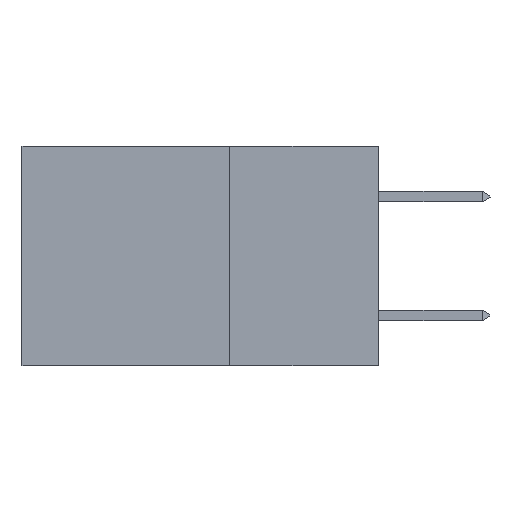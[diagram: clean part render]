
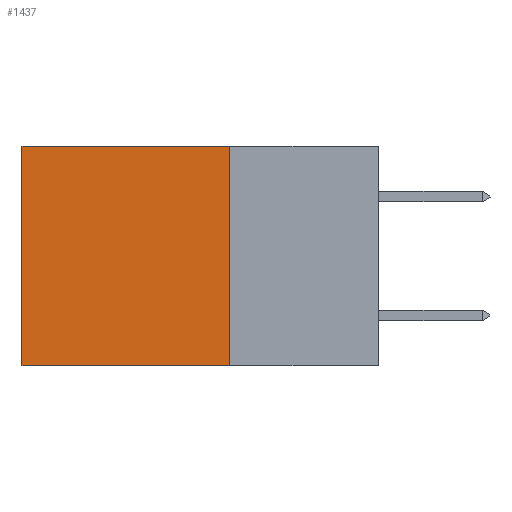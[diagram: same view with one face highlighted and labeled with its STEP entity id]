
A CAD part, left-side view. The second image highlights one B-rep face of the part: STEP entity #1437.
In plain terms, the highlighted planar face has unit normal (-1, 0, 0).
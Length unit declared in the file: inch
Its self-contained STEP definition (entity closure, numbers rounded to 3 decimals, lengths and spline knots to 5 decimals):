
#185 = CARTESIAN_POINT ( 'NONE',  ( 0.298, 0.25, -0.37 ) ) ;
#288 = EDGE_LOOP ( 'NONE', ( #7681, #10519, #3597, #2928 ) ) ;
#947 = DIRECTION ( 'NONE',  ( 1., 0., 0. ) ) ;
#1437 = ADVANCED_FACE ( 'NONE', ( #12549 ), #7735, .F. ) ;
#1477 = EDGE_CURVE ( 'NONE', #9603, #2144, #6084, .T. ) ;
#2076 = CARTESIAN_POINT ( 'NONE',  ( 0.298, 0.25, 0. ) ) ;
#2144 = VERTEX_POINT ( 'NONE', #185 ) ;
#2149 = EDGE_CURVE ( 'NONE', #2144, #10290, #9883, .T. ) ;
#2884 = CARTESIAN_POINT ( 'NONE',  ( 0.298, 0.6, 0. ) ) ;
#2928 = ORIENTED_EDGE ( 'NONE', *, *, #3983, .T. ) ;
#2933 = CARTESIAN_POINT ( 'NONE',  ( 0.298, 0.6, 0. ) ) ;
#3207 = DIRECTION ( 'NONE',  ( 0., 0., -1. ) ) ;
#3597 = ORIENTED_EDGE ( 'NONE', *, *, #1477, .F. ) ;
#3614 = CARTESIAN_POINT ( 'NONE',  ( 0.298, 0.25, 0. ) ) ;
#3936 = VECTOR ( 'NONE', #12483, 39.37008 ) ;
#3954 = CARTESIAN_POINT ( 'NONE',  ( 0.298, 0.6, -0.37 ) ) ;
#3983 = EDGE_CURVE ( 'NONE', #9603, #10098, #11292, .T. ) ;
#4499 = VECTOR ( 'NONE', #12167, 39.37008 ) ;
#4834 = VECTOR ( 'NONE', #7199, 39.37008 ) ;
#5842 = CARTESIAN_POINT ( 'NONE',  ( 0.298, 0.25, -0.37 ) ) ;
#5880 = DIRECTION ( 'NONE',  ( 0., 1., 0. ) ) ;
#6084 = LINE ( 'NONE', #2076, #4499 ) ;
#6552 = CARTESIAN_POINT ( 'NONE',  ( 0.298, 0.25, 0. ) ) ;
#7199 = DIRECTION ( 'NONE',  ( 0., 0., -1. ) ) ;
#7681 = ORIENTED_EDGE ( 'NONE', *, *, #10935, .T. ) ;
#7735 = PLANE ( 'NONE',  #9898 ) ;
#7775 = CARTESIAN_POINT ( 'NONE',  ( 0.298, 0.25, 0. ) ) ;
#9603 = VERTEX_POINT ( 'NONE', #7775 ) ;
#9883 = LINE ( 'NONE', #5842, #3936 ) ;
#9898 = AXIS2_PLACEMENT_3D ( 'NONE', #6552, #947, #3207 ) ;
#10098 = VERTEX_POINT ( 'NONE', #2884 ) ;
#10290 = VERTEX_POINT ( 'NONE', #3954 ) ;
#10519 = ORIENTED_EDGE ( 'NONE', *, *, #2149, .F. ) ;
#10935 = EDGE_CURVE ( 'NONE', #10098, #10290, #13572, .T. ) ;
#11292 = LINE ( 'NONE', #3614, #13882 ) ;
#12167 = DIRECTION ( 'NONE',  ( 0., 0., -1. ) ) ;
#12483 = DIRECTION ( 'NONE',  ( 0., 1., 0. ) ) ;
#12549 = FACE_OUTER_BOUND ( 'NONE', #288, .T. ) ;
#13572 = LINE ( 'NONE', #2933, #4834 ) ;
#13882 = VECTOR ( 'NONE', #5880, 39.37008 ) ;
